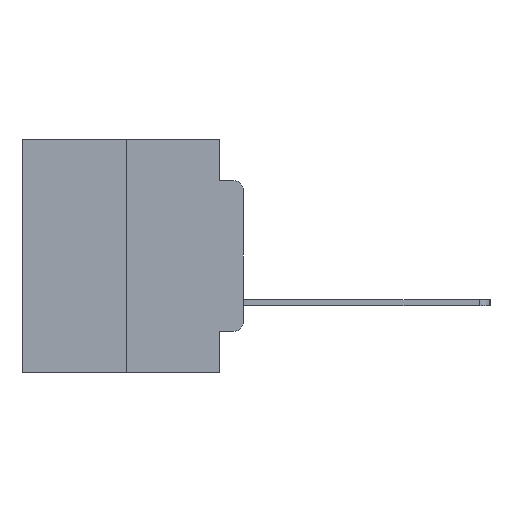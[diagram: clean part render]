
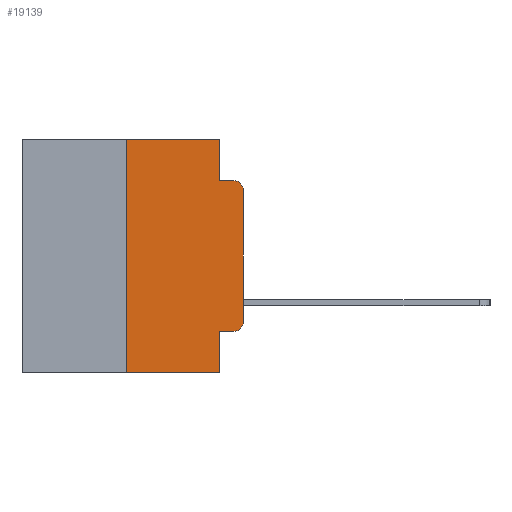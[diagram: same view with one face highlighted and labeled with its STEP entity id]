
A CAD part, left-side view. The second image highlights one B-rep face of the part: STEP entity #19139.
In plain terms, the highlighted planar face has unit normal (-1, 0, 0).
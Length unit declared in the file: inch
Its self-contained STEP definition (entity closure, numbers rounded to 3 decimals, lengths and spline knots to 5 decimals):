
#259 = VECTOR ( 'NONE', #9537, 39.37008 ) ;
#622 = LINE ( 'NONE', #21086, #10887 ) ;
#1167 = DIRECTION ( 'NONE',  ( 0., 0., -1. ) ) ;
#2110 = EDGE_CURVE ( 'NONE', #18885, #22702, #22310, .T. ) ;
#2609 = DIRECTION ( 'NONE',  ( 0., 0., -1. ) ) ;
#2828 = DIRECTION ( 'NONE',  ( 0., -1., 0. ) ) ;
#3136 = CARTESIAN_POINT ( 'NONE',  ( 0., 0.25, -0.5 ) ) ;
#3238 = VERTEX_POINT ( 'NONE', #11994 ) ;
#3298 = CARTESIAN_POINT ( 'NONE',  ( 0., 0.051, 0. ) ) ;
#4590 = CARTESIAN_POINT ( 'NONE',  ( 0., 0.051, -0.4115 ) ) ;
#4979 = VERTEX_POINT ( 'NONE', #19910 ) ;
#5486 = CARTESIAN_POINT ( 'NONE',  ( 0., 0.02, -0.0885 ) ) ;
#5745 = VECTOR ( 'NONE', #2609, 39.37008 ) ;
#5851 = LINE ( 'NONE', #9468, #259 ) ;
#6349 = EDGE_CURVE ( 'NONE', #3238, #4979, #11675, .T. ) ;
#6383 = ORIENTED_EDGE ( 'NONE', *, *, #6349, .F. ) ;
#6867 = VECTOR ( 'NONE', #11057, 39.37008 ) ;
#6949 = FACE_OUTER_BOUND ( 'NONE', #23262, .T. ) ;
#7354 = ORIENTED_EDGE ( 'NONE', *, *, #16801, .T. ) ;
#7412 = DIRECTION ( 'NONE',  ( 0., 0., -1. ) ) ;
#8284 = ORIENTED_EDGE ( 'NONE', *, *, #12332, .T. ) ;
#8839 = CARTESIAN_POINT ( 'NONE',  ( 0., 0.051, 0. ) ) ;
#8917 = CARTESIAN_POINT ( 'NONE',  ( 0., 0., -0.3915 ) ) ;
#9468 = CARTESIAN_POINT ( 'NONE',  ( 0., 0.473, 0. ) ) ;
#9537 = DIRECTION ( 'NONE',  ( 0., -1., 0. ) ) ;
#10426 = DIRECTION ( 'NONE',  ( 0., -1., 0. ) ) ;
#10771 = CARTESIAN_POINT ( 'NONE',  ( 0., 0.02, -0.1085 ) ) ;
#10887 = VECTOR ( 'NONE', #22954, 39.37008 ) ;
#10975 = CIRCLE ( 'NONE', #23641, 0.02 ) ;
#11057 = DIRECTION ( 'NONE',  ( 0., 0., 1. ) ) ;
#11669 = ORIENTED_EDGE ( 'NONE', *, *, #12976, .F. ) ;
#11675 = LINE ( 'NONE', #8839, #5745 ) ;
#11964 = CARTESIAN_POINT ( 'NONE',  ( 0., 0.473, 0. ) ) ;
#11994 = CARTESIAN_POINT ( 'NONE',  ( 0., 0.051, 0. ) ) ;
#12143 = VERTEX_POINT ( 'NONE', #8917 ) ;
#12179 = VECTOR ( 'NONE', #20606, 39.37008 ) ;
#12326 = VECTOR ( 'NONE', #2828, 39.37008 ) ;
#12332 = EDGE_CURVE ( 'NONE', #18885, #14201, #622, .T. ) ;
#12734 = DIRECTION ( 'NONE',  ( 0., 0., -1. ) ) ;
#12976 = EDGE_CURVE ( 'NONE', #4979, #13175, #22446, .T. ) ;
#13106 = CARTESIAN_POINT ( 'NONE',  ( 0., 0., 0. ) ) ;
#13175 = VERTEX_POINT ( 'NONE', #5486 ) ;
#13302 = DIRECTION ( 'NONE',  ( -1., 0., 0. ) ) ;
#13363 = VERTEX_POINT ( 'NONE', #15955 ) ;
#13482 = ORIENTED_EDGE ( 'NONE', *, *, #2110, .F. ) ;
#13779 = ORIENTED_EDGE ( 'NONE', *, *, #15532, .T. ) ;
#13906 = DIRECTION ( 'NONE',  ( 0., 0., -1. ) ) ;
#14160 = CARTESIAN_POINT ( 'NONE',  ( 0., 0.051, -0.4115 ) ) ;
#14201 = VERTEX_POINT ( 'NONE', #15415 ) ;
#14347 = CIRCLE ( 'NONE', #14448, 0.02 ) ;
#14448 = AXIS2_PLACEMENT_3D ( 'NONE', #24639, #13302, #1167 ) ;
#14511 = VERTEX_POINT ( 'NONE', #4590 ) ;
#14733 = EDGE_CURVE ( 'NONE', #15638, #12143, #14347, .T. ) ;
#14960 = LINE ( 'NONE', #3298, #23819 ) ;
#15415 = CARTESIAN_POINT ( 'NONE',  ( 0., 0.051, -0.5 ) ) ;
#15532 = EDGE_CURVE ( 'NONE', #13363, #13175, #10975, .T. ) ;
#15638 = VERTEX_POINT ( 'NONE', #16819 ) ;
#15955 = CARTESIAN_POINT ( 'NONE',  ( 0., 0., -0.1085 ) ) ;
#16801 = EDGE_CURVE ( 'NONE', #12143, #13363, #22245, .T. ) ;
#16819 = CARTESIAN_POINT ( 'NONE',  ( 0., 0.02, -0.4115 ) ) ;
#16868 = VECTOR ( 'NONE', #10426, 39.37008 ) ;
#17228 = AXIS2_PLACEMENT_3D ( 'NONE', #11964, #25246, #13906 ) ;
#17399 = CARTESIAN_POINT ( 'NONE',  ( 0., 0.25, 0. ) ) ;
#17688 = PLANE ( 'NONE',  #17228 ) ;
#18208 = EDGE_CURVE ( 'NONE', #22702, #3238, #5851, .T. ) ;
#18298 = CARTESIAN_POINT ( 'NONE',  ( 0., 0.25, 0. ) ) ;
#18513 = CARTESIAN_POINT ( 'NONE',  ( 0., 0.051, -0.0885 ) ) ;
#18885 = VERTEX_POINT ( 'NONE', #3136 ) ;
#19139 = ADVANCED_FACE ( 'NONE', ( #6949 ), #17688, .F. ) ;
#19910 = CARTESIAN_POINT ( 'NONE',  ( 0., 0.051, -0.0885 ) ) ;
#20606 = DIRECTION ( 'NONE',  ( 0., 0., 1. ) ) ;
#20956 = ORIENTED_EDGE ( 'NONE', *, *, #14733, .T. ) ;
#21086 = CARTESIAN_POINT ( 'NONE',  ( 0., 0.473, -0.5 ) ) ;
#21117 = EDGE_CURVE ( 'NONE', #14511, #15638, #22486, .T. ) ;
#21965 = ORIENTED_EDGE ( 'NONE', *, *, #21117, .T. ) ;
#22245 = LINE ( 'NONE', #13106, #6867 ) ;
#22310 = LINE ( 'NONE', #17399, #12179 ) ;
#22446 = LINE ( 'NONE', #18513, #12326 ) ;
#22486 = LINE ( 'NONE', #14160, #16868 ) ;
#22702 = VERTEX_POINT ( 'NONE', #18298 ) ;
#22954 = DIRECTION ( 'NONE',  ( 0., -1., 0. ) ) ;
#22978 = ORIENTED_EDGE ( 'NONE', *, *, #18208, .F. ) ;
#23262 = EDGE_LOOP ( 'NONE', ( #7354, #13779, #11669, #6383, #22978, #13482, #8284, #24150, #21965, #20956 ) ) ;
#23600 = EDGE_CURVE ( 'NONE', #14511, #14201, #14960, .T. ) ;
#23641 = AXIS2_PLACEMENT_3D ( 'NONE', #10771, #24093, #12734 ) ;
#23819 = VECTOR ( 'NONE', #7412, 39.37008 ) ;
#24093 = DIRECTION ( 'NONE',  ( -1., 0., 0. ) ) ;
#24150 = ORIENTED_EDGE ( 'NONE', *, *, #23600, .F. ) ;
#24639 = CARTESIAN_POINT ( 'NONE',  ( 0., 0.02, -0.3915 ) ) ;
#25246 = DIRECTION ( 'NONE',  ( 1., 0., 0. ) ) ;
